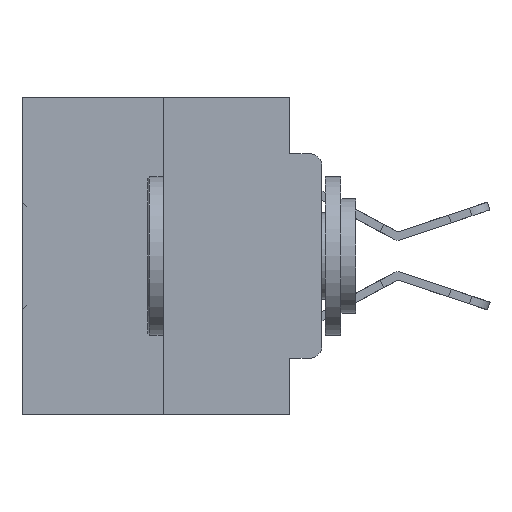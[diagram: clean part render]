
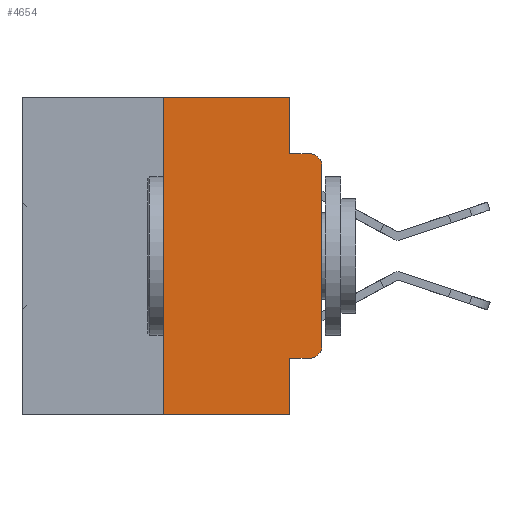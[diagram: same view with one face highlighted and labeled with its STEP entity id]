
A CAD part, left-side view. The second image highlights one B-rep face of the part: STEP entity #4654.
In plain terms, the highlighted planar face has unit normal (-1, 0, 0).
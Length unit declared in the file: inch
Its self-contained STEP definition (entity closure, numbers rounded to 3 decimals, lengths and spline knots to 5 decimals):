
#679 = CARTESIAN_POINT ( 'NONE',  ( 0., 0.473, -0.5 ) ) ;
#930 = ORIENTED_EDGE ( 'NONE', *, *, #8127, .T. ) ;
#1794 = VECTOR ( 'NONE', #34295, 39.37008 ) ;
#1980 = CARTESIAN_POINT ( 'NONE',  ( 0., 0.25, -0.5 ) ) ;
#2072 = LINE ( 'NONE', #4917, #8345 ) ;
#2739 = VECTOR ( 'NONE', #31107, 39.37008 ) ;
#2970 = ORIENTED_EDGE ( 'NONE', *, *, #19276, .F. ) ;
#3251 = DIRECTION ( 'NONE',  ( 0., 0., 1. ) ) ;
#4588 = VERTEX_POINT ( 'NONE', #15993 ) ;
#4654 = ADVANCED_FACE ( 'NONE', ( #25029 ), #22012, .F. ) ;
#4917 = CARTESIAN_POINT ( 'NONE',  ( 0., 0.25, 0. ) ) ;
#4950 = VERTEX_POINT ( 'NONE', #8252 ) ;
#5060 = LINE ( 'NONE', #6265, #30733 ) ;
#5486 = DIRECTION ( 'NONE',  ( 0., 0., -1. ) ) ;
#5589 = CARTESIAN_POINT ( 'NONE',  ( 0., 0.02, -0.3915 ) ) ;
#6265 = CARTESIAN_POINT ( 'NONE',  ( 0., 0., 0. ) ) ;
#6749 = CARTESIAN_POINT ( 'NONE',  ( 0., 0.051, -0.4115 ) ) ;
#6965 = CARTESIAN_POINT ( 'NONE',  ( 0., 0.473, 0. ) ) ;
#7454 = ORIENTED_EDGE ( 'NONE', *, *, #31440, .F. ) ;
#8117 = AXIS2_PLACEMENT_3D ( 'NONE', #5589, #16435, #24432 ) ;
#8127 = EDGE_CURVE ( 'NONE', #9061, #25703, #18879, .T. ) ;
#8165 = CARTESIAN_POINT ( 'NONE',  ( 0., 0.25, 0. ) ) ;
#8252 = CARTESIAN_POINT ( 'NONE',  ( 0., 0., -0.1085 ) ) ;
#8345 = VECTOR ( 'NONE', #30332, 39.37008 ) ;
#9061 = VERTEX_POINT ( 'NONE', #22802 ) ;
#10171 = LINE ( 'NONE', #6965, #27803 ) ;
#10855 = ORIENTED_EDGE ( 'NONE', *, *, #11992, .F. ) ;
#10898 = DIRECTION ( 'NONE',  ( 0., -1., 0. ) ) ;
#11449 = AXIS2_PLACEMENT_3D ( 'NONE', #15770, #21629, #29476 ) ;
#11992 = EDGE_CURVE ( 'NONE', #26095, #24480, #27411, .T. ) ;
#12261 = LINE ( 'NONE', #28442, #1794 ) ;
#12456 = LINE ( 'NONE', #28097, #24205 ) ;
#13044 = CARTESIAN_POINT ( 'NONE',  ( 0., 0.051, 0. ) ) ;
#14206 = DIRECTION ( 'NONE',  ( 1., 0., 0. ) ) ;
#14340 = VERTEX_POINT ( 'NONE', #13044 ) ;
#15770 = CARTESIAN_POINT ( 'NONE',  ( 0., 0.02, -0.1085 ) ) ;
#15993 = CARTESIAN_POINT ( 'NONE',  ( 0., 0.051, -0.4115 ) ) ;
#16000 = VECTOR ( 'NONE', #20424, 39.37008 ) ;
#16124 = CARTESIAN_POINT ( 'NONE',  ( 0., 0., -0.3915 ) ) ;
#16435 = DIRECTION ( 'NONE',  ( -1., 0., 0. ) ) ;
#17549 = EDGE_CURVE ( 'NONE', #25171, #14340, #10171, .T. ) ;
#17789 = DIRECTION ( 'NONE',  ( 0., -1., 0. ) ) ;
#18879 = CIRCLE ( 'NONE', #8117, 0.02 ) ;
#18911 = CARTESIAN_POINT ( 'NONE',  ( 0., 0.051, -0.0885 ) ) ;
#19276 = EDGE_CURVE ( 'NONE', #4588, #19707, #12261, .T. ) ;
#19307 = EDGE_CURVE ( 'NONE', #4588, #9061, #31125, .T. ) ;
#19627 = CARTESIAN_POINT ( 'NONE',  ( 0., 0.051, -0.5 ) ) ;
#19707 = VERTEX_POINT ( 'NONE', #19627 ) ;
#19900 = DIRECTION ( 'NONE',  ( 0., 0., -1. ) ) ;
#20077 = EDGE_CURVE ( 'NONE', #25703, #4950, #5060, .T. ) ;
#20424 = DIRECTION ( 'NONE',  ( 0., -1., 0. ) ) ;
#21629 = DIRECTION ( 'NONE',  ( -1., 0., 0. ) ) ;
#22012 = PLANE ( 'NONE',  #32445 ) ;
#22182 = ORIENTED_EDGE ( 'NONE', *, *, #34224, .T. ) ;
#22802 = CARTESIAN_POINT ( 'NONE',  ( 0., 0.02, -0.4115 ) ) ;
#22891 = LINE ( 'NONE', #679, #2739 ) ;
#23793 = ORIENTED_EDGE ( 'NONE', *, *, #30825, .F. ) ;
#24205 = VECTOR ( 'NONE', #19900, 39.37008 ) ;
#24208 = EDGE_CURVE ( 'NONE', #4950, #24480, #26795, .T. ) ;
#24432 = DIRECTION ( 'NONE',  ( 0., 0., -1. ) ) ;
#24480 = VERTEX_POINT ( 'NONE', #28547 ) ;
#24879 = ORIENTED_EDGE ( 'NONE', *, *, #20077, .T. ) ;
#25029 = FACE_OUTER_BOUND ( 'NONE', #33440, .T. ) ;
#25171 = VERTEX_POINT ( 'NONE', #8165 ) ;
#25703 = VERTEX_POINT ( 'NONE', #16124 ) ;
#25896 = VECTOR ( 'NONE', #10898, 39.37008 ) ;
#26095 = VERTEX_POINT ( 'NONE', #18911 ) ;
#26795 = CIRCLE ( 'NONE', #11449, 0.02 ) ;
#27411 = LINE ( 'NONE', #33098, #25896 ) ;
#27803 = VECTOR ( 'NONE', #17789, 39.37008 ) ;
#28097 = CARTESIAN_POINT ( 'NONE',  ( 0., 0.051, 0. ) ) ;
#28222 = VERTEX_POINT ( 'NONE', #1980 ) ;
#28442 = CARTESIAN_POINT ( 'NONE',  ( 0., 0.051, 0. ) ) ;
#28477 = ORIENTED_EDGE ( 'NONE', *, *, #17549, .F. ) ;
#28547 = CARTESIAN_POINT ( 'NONE',  ( 0., 0.02, -0.0885 ) ) ;
#29476 = DIRECTION ( 'NONE',  ( 0., 0., -1. ) ) ;
#30332 = DIRECTION ( 'NONE',  ( 0., 0., 1. ) ) ;
#30733 = VECTOR ( 'NONE', #3251, 39.37008 ) ;
#30825 = EDGE_CURVE ( 'NONE', #14340, #26095, #12456, .T. ) ;
#31075 = ORIENTED_EDGE ( 'NONE', *, *, #19307, .T. ) ;
#31107 = DIRECTION ( 'NONE',  ( 0., -1., 0. ) ) ;
#31125 = LINE ( 'NONE', #6749, #16000 ) ;
#31440 = EDGE_CURVE ( 'NONE', #28222, #25171, #2072, .T. ) ;
#32445 = AXIS2_PLACEMENT_3D ( 'NONE', #33044, #14206, #5486 ) ;
#33044 = CARTESIAN_POINT ( 'NONE',  ( 0., 0.473, 0. ) ) ;
#33098 = CARTESIAN_POINT ( 'NONE',  ( 0., 0.051, -0.0885 ) ) ;
#33185 = ORIENTED_EDGE ( 'NONE', *, *, #24208, .T. ) ;
#33440 = EDGE_LOOP ( 'NONE', ( #24879, #33185, #10855, #23793, #28477, #7454, #22182, #2970, #31075, #930 ) ) ;
#34224 = EDGE_CURVE ( 'NONE', #28222, #19707, #22891, .T. ) ;
#34295 = DIRECTION ( 'NONE',  ( 0., 0., -1. ) ) ;
